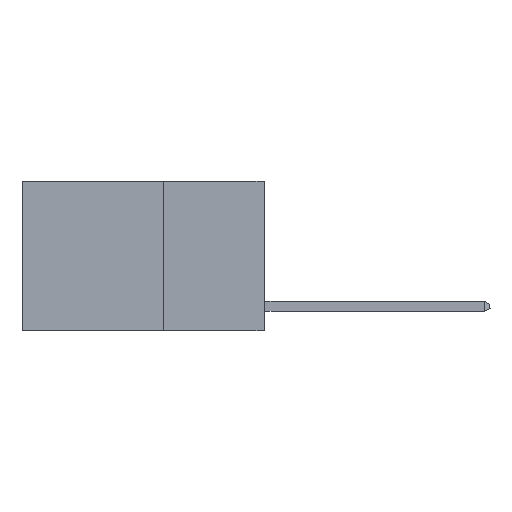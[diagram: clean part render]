
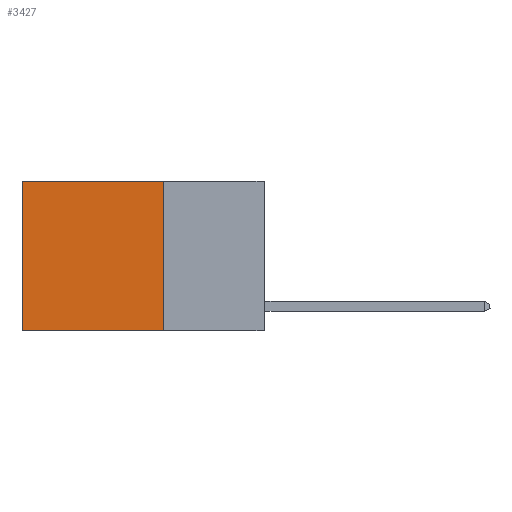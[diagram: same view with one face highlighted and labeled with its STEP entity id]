
A CAD part, left-side view. The second image highlights one B-rep face of the part: STEP entity #3427.
In plain terms, the highlighted planar face has unit normal (-1, 0, 0).
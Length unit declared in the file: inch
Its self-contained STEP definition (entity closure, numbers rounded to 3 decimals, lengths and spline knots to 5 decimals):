
#94 = VERTEX_POINT ( 'NONE', #5774 ) ;
#161 = DIRECTION ( 'NONE',  ( 0., 0., -1. ) ) ;
#1823 = VECTOR ( 'NONE', #4210, 39.37008 ) ;
#2124 = EDGE_CURVE ( 'NONE', #17930, #11472, #12551, .T. ) ;
#2344 = ORIENTED_EDGE ( 'NONE', *, *, #18111, .F. ) ;
#3427 = ADVANCED_FACE ( 'NONE', ( #18509 ), #20478, .F. ) ;
#3445 = LINE ( 'NONE', #17608, #12482 ) ;
#4210 = DIRECTION ( 'NONE',  ( 0., 1., 0. ) ) ;
#4468 = ORIENTED_EDGE ( 'NONE', *, *, #2124, .F. ) ;
#5774 = CARTESIAN_POINT ( 'NONE',  ( 0.2625, 0.6, -0.37 ) ) ;
#7595 = CARTESIAN_POINT ( 'NONE',  ( 0.2625, 0.25, -0.37 ) ) ;
#8566 = CARTESIAN_POINT ( 'NONE',  ( 0.2625, 0.25, 0. ) ) ;
#8841 = CARTESIAN_POINT ( 'NONE',  ( 0.2625, 0.25, 0. ) ) ;
#9200 = DIRECTION ( 'NONE',  ( 0., 0., -1. ) ) ;
#9225 = ORIENTED_EDGE ( 'NONE', *, *, #18077, .T. ) ;
#10451 = DIRECTION ( 'NONE',  ( 1., 0., 0. ) ) ;
#10772 = ORIENTED_EDGE ( 'NONE', *, *, #14472, .T. ) ;
#10999 = EDGE_LOOP ( 'NONE', ( #9225, #2344, #4468, #10772 ) ) ;
#11046 = AXIS2_PLACEMENT_3D ( 'NONE', #12084, #10451, #161 ) ;
#11472 = VERTEX_POINT ( 'NONE', #7595 ) ;
#11503 = VERTEX_POINT ( 'NONE', #16075 ) ;
#12018 = VECTOR ( 'NONE', #13680, 39.37008 ) ;
#12084 = CARTESIAN_POINT ( 'NONE',  ( 0.2625, 0.25, 0. ) ) ;
#12342 = VECTOR ( 'NONE', #18697, 39.37008 ) ;
#12482 = VECTOR ( 'NONE', #9200, 39.37008 ) ;
#12551 = LINE ( 'NONE', #8566, #12018 ) ;
#12877 = LINE ( 'NONE', #20372, #12342 ) ;
#13680 = DIRECTION ( 'NONE',  ( 0., 0., -1. ) ) ;
#14371 = CARTESIAN_POINT ( 'NONE',  ( 0.2625, 0.25, -0.37 ) ) ;
#14472 = EDGE_CURVE ( 'NONE', #17930, #11503, #12877, .T. ) ;
#16075 = CARTESIAN_POINT ( 'NONE',  ( 0.2625, 0.6, 0. ) ) ;
#17608 = CARTESIAN_POINT ( 'NONE',  ( 0.2625, 0.6, 0. ) ) ;
#17930 = VERTEX_POINT ( 'NONE', #8841 ) ;
#18077 = EDGE_CURVE ( 'NONE', #11503, #94, #3445, .T. ) ;
#18111 = EDGE_CURVE ( 'NONE', #11472, #94, #19248, .T. ) ;
#18509 = FACE_OUTER_BOUND ( 'NONE', #10999, .T. ) ;
#18697 = DIRECTION ( 'NONE',  ( 0., 1., 0. ) ) ;
#19248 = LINE ( 'NONE', #14371, #1823 ) ;
#20372 = CARTESIAN_POINT ( 'NONE',  ( 0.2625, 0.25, 0. ) ) ;
#20478 = PLANE ( 'NONE',  #11046 ) ;
